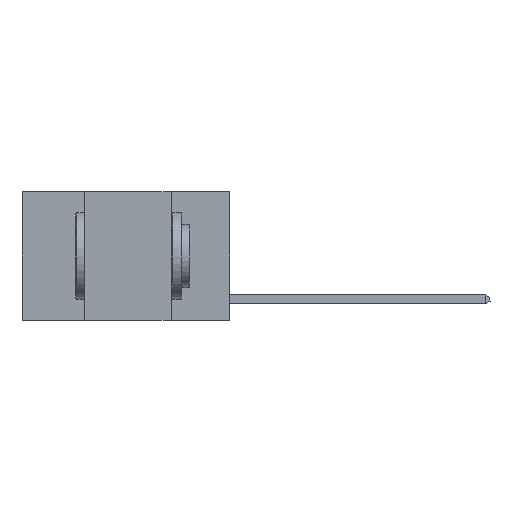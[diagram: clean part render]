
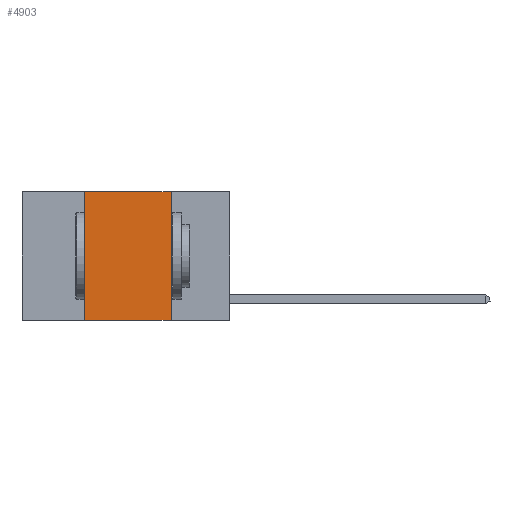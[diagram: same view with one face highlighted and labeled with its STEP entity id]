
A CAD part, left-side view. The second image highlights one B-rep face of the part: STEP entity #4903.
In plain terms, the highlighted planar face has unit normal (-1, 0, 0).
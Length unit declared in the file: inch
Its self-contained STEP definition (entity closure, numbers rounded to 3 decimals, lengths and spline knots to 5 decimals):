
#111 = LINE ( 'NONE', #5708, #17073 ) ;
#491 = CARTESIAN_POINT ( 'NONE',  ( 0., 0.6, 0. ) ) ;
#1755 = CARTESIAN_POINT ( 'NONE',  ( 0., 0.17, 0. ) ) ;
#1916 = AXIS2_PLACEMENT_3D ( 'NONE', #5583, #5773, #8795 ) ;
#1939 = VECTOR ( 'NONE', #10514, 39.37008 ) ;
#1964 = LINE ( 'NONE', #491, #6426 ) ;
#2231 = ORIENTED_EDGE ( 'NONE', *, *, #12716, .F. ) ;
#2363 = EDGE_LOOP ( 'NONE', ( #2231, #13466, #16202, #3204 ) ) ;
#2391 = EDGE_CURVE ( 'NONE', #6128, #12091, #1964, .T. ) ;
#2547 = CARTESIAN_POINT ( 'NONE',  ( 0., 0.42, -0.37 ) ) ;
#3062 = CARTESIAN_POINT ( 'NONE',  ( 0., 0.6, -0.37 ) ) ;
#3204 = ORIENTED_EDGE ( 'NONE', *, *, #12004, .T. ) ;
#4358 = VERTEX_POINT ( 'NONE', #7288 ) ;
#4613 = LINE ( 'NONE', #13250, #1939 ) ;
#4903 = ADVANCED_FACE ( 'NONE', ( #16969 ), #11614, .F. ) ;
#5583 = CARTESIAN_POINT ( 'NONE',  ( 0., 0.6, 0. ) ) ;
#5708 = CARTESIAN_POINT ( 'NONE',  ( 0., 0.17, 0. ) ) ;
#5773 = DIRECTION ( 'NONE',  ( 1., 0., 0. ) ) ;
#5859 = EDGE_CURVE ( 'NONE', #10892, #6128, #4613, .T. ) ;
#6128 = VERTEX_POINT ( 'NONE', #7015 ) ;
#6269 = VECTOR ( 'NONE', #11897, 39.37008 ) ;
#6426 = VECTOR ( 'NONE', #13599, 39.37008 ) ;
#7015 = CARTESIAN_POINT ( 'NONE',  ( 0., 0.42, 0. ) ) ;
#7035 = DIRECTION ( 'NONE',  ( 0., 0., -1. ) ) ;
#7288 = CARTESIAN_POINT ( 'NONE',  ( 0., 0.17, -0.37 ) ) ;
#7666 = LINE ( 'NONE', #3062, #6269 ) ;
#8795 = DIRECTION ( 'NONE',  ( 0., 0., -1. ) ) ;
#10514 = DIRECTION ( 'NONE',  ( 0., 0., 1. ) ) ;
#10892 = VERTEX_POINT ( 'NONE', #2547 ) ;
#11614 = PLANE ( 'NONE',  #1916 ) ;
#11897 = DIRECTION ( 'NONE',  ( 0., -1., 0. ) ) ;
#12004 = EDGE_CURVE ( 'NONE', #10892, #4358, #7666, .T. ) ;
#12091 = VERTEX_POINT ( 'NONE', #1755 ) ;
#12716 = EDGE_CURVE ( 'NONE', #12091, #4358, #111, .T. ) ;
#13250 = CARTESIAN_POINT ( 'NONE',  ( 0., 0.42, 0. ) ) ;
#13466 = ORIENTED_EDGE ( 'NONE', *, *, #2391, .F. ) ;
#13599 = DIRECTION ( 'NONE',  ( 0., -1., 0. ) ) ;
#16202 = ORIENTED_EDGE ( 'NONE', *, *, #5859, .F. ) ;
#16969 = FACE_OUTER_BOUND ( 'NONE', #2363, .T. ) ;
#17073 = VECTOR ( 'NONE', #7035, 39.37008 ) ;
